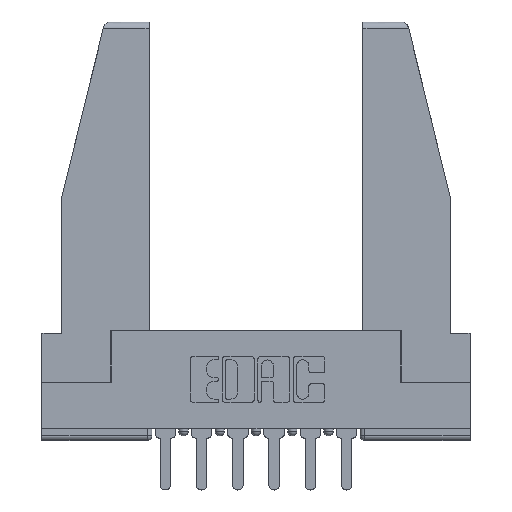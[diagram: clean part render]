
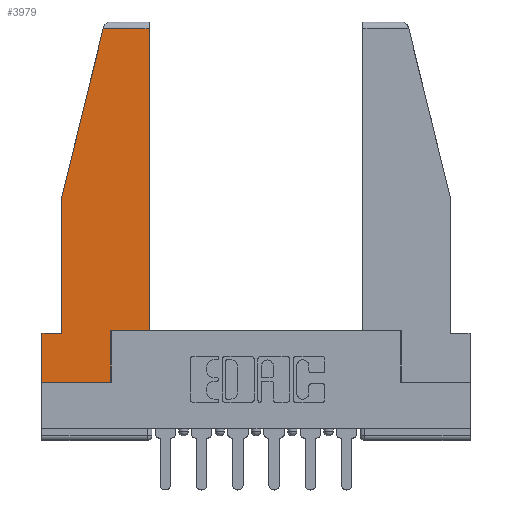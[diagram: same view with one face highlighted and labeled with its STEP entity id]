
A CAD part, top view. The second image highlights one B-rep face of the part: STEP entity #3979.
In plain terms, the highlighted planar face has unit normal (0, 0, 1).
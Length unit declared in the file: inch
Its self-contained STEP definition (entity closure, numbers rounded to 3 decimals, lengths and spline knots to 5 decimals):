
#81 = VERTEX_POINT ( 'NONE', #7556 ) ;
#235 = DIRECTION ( 'NONE',  ( 0., -1., 0. ) ) ;
#490 = LINE ( 'NONE', #7097, #2949 ) ;
#555 = CARTESIAN_POINT ( 'NONE',  ( 0.271, 1.55, 0. ) ) ;
#639 = CARTESIAN_POINT ( 'NONE',  ( 0.461, 1.52, 0. ) ) ;
#874 = EDGE_CURVE ( 'NONE', #11255, #3614, #11447, .T. ) ;
#1006 = ORIENTED_EDGE ( 'NONE', *, *, #5677, .T. ) ;
#1264 = CARTESIAN_POINT ( 'NONE',  ( 0.297, 0.223, 0. ) ) ;
#1443 = EDGE_CURVE ( 'NONE', #4556, #1515, #490, .T. ) ;
#1515 = VERTEX_POINT ( 'NONE', #9758 ) ;
#2089 = LINE ( 'NONE', #5869, #9575 ) ;
#2135 = ORIENTED_EDGE ( 'NONE', *, *, #4913, .T. ) ;
#2151 = VERTEX_POINT ( 'NONE', #10911 ) ;
#2249 = EDGE_CURVE ( 'NONE', #2151, #4882, #11339, .T. ) ;
#2949 = VECTOR ( 'NONE', #6114, 39.37008 ) ;
#2973 = FACE_OUTER_BOUND ( 'NONE', #5602, .T. ) ;
#3452 = CARTESIAN_POINT ( 'NONE',  ( 0.297, 0., 0. ) ) ;
#3614 = VERTEX_POINT ( 'NONE', #4164 ) ;
#3716 = ORIENTED_EDGE ( 'NONE', *, *, #8319, .T. ) ;
#3979 = ADVANCED_FACE ( 'NONE', ( #2973 ), #6754, .T. ) ;
#4010 = DIRECTION ( 'NONE',  ( -1., 0., 0. ) ) ;
#4101 = EDGE_CURVE ( 'NONE', #3614, #9369, #4502, .T. ) ;
#4164 = CARTESIAN_POINT ( 'NONE',  ( 0.297, 0., 0. ) ) ;
#4388 = VECTOR ( 'NONE', #10184, 39.37008 ) ;
#4502 = LINE ( 'NONE', #3452, #4388 ) ;
#4556 = VERTEX_POINT ( 'NONE', #639 ) ;
#4742 = ORIENTED_EDGE ( 'NONE', *, *, #8658, .T. ) ;
#4882 = VERTEX_POINT ( 'NONE', #7933 ) ;
#4913 = EDGE_CURVE ( 'NONE', #9369, #81, #5036, .T. ) ;
#4996 = CARTESIAN_POINT ( 'NONE',  ( 0., 0.21, 0. ) ) ;
#5036 = LINE ( 'NONE', #1264, #8338 ) ;
#5232 = CARTESIAN_POINT ( 'NONE',  ( 0.461, 0.223, 0. ) ) ;
#5293 = LINE ( 'NONE', #5232, #8551 ) ;
#5384 = ORIENTED_EDGE ( 'NONE', *, *, #2249, .T. ) ;
#5568 = DIRECTION ( 'NONE',  ( 0., 0., 1. ) ) ;
#5602 = EDGE_LOOP ( 'NONE', ( #1006, #5768, #3716, #5384, #4742, #7969, #5759, #8676, #2135 ) ) ;
#5677 = EDGE_CURVE ( 'NONE', #81, #4556, #5293, .T. ) ;
#5759 = ORIENTED_EDGE ( 'NONE', *, *, #874, .T. ) ;
#5768 = ORIENTED_EDGE ( 'NONE', *, *, #1443, .T. ) ;
#5784 = VECTOR ( 'NONE', #4010, 39.37008 ) ;
#5869 = CARTESIAN_POINT ( 'NONE',  ( 0., 0.21, 0. ) ) ;
#6114 = DIRECTION ( 'NONE',  ( -1., 0., 0. ) ) ;
#6341 = DIRECTION ( 'NONE',  ( 0., 1., 0. ) ) ;
#6673 = VECTOR ( 'NONE', #10585, 39.37008 ) ;
#6754 = PLANE ( 'NONE',  #10698 ) ;
#6773 = VECTOR ( 'NONE', #7278, 39.37008 ) ;
#7097 = CARTESIAN_POINT ( 'NONE',  ( 0., 1.52, 0. ) ) ;
#7278 = DIRECTION ( 'NONE',  ( -0.239, -0.971, 0. ) ) ;
#7556 = CARTESIAN_POINT ( 'NONE',  ( 0.461, 0.223, 0. ) ) ;
#7669 = CARTESIAN_POINT ( 'NONE',  ( 0., 0., 0. ) ) ;
#7713 = LINE ( 'NONE', #8689, #5784 ) ;
#7933 = CARTESIAN_POINT ( 'NONE',  ( 0.086, 0.21, 0. ) ) ;
#7969 = ORIENTED_EDGE ( 'NONE', *, *, #11056, .T. ) ;
#8082 = VECTOR ( 'NONE', #9461, 39.37008 ) ;
#8135 = LINE ( 'NONE', #555, #6773 ) ;
#8319 = EDGE_CURVE ( 'NONE', #1515, #2151, #8135, .T. ) ;
#8338 = VECTOR ( 'NONE', #8851, 39.37008 ) ;
#8401 = DIRECTION ( 'NONE',  ( 1., 0., 0. ) ) ;
#8551 = VECTOR ( 'NONE', #6341, 39.37008 ) ;
#8658 = EDGE_CURVE ( 'NONE', #4882, #11010, #7713, .T. ) ;
#8676 = ORIENTED_EDGE ( 'NONE', *, *, #4101, .T. ) ;
#8689 = CARTESIAN_POINT ( 'NONE',  ( 0., 0.21, 0. ) ) ;
#8851 = DIRECTION ( 'NONE',  ( 1., 0., 0. ) ) ;
#9369 = VERTEX_POINT ( 'NONE', #11744 ) ;
#9461 = DIRECTION ( 'NONE',  ( 0., -1., 0. ) ) ;
#9575 = VECTOR ( 'NONE', #235, 39.37008 ) ;
#9758 = CARTESIAN_POINT ( 'NONE',  ( 0.2636, 1.52, 0. ) ) ;
#10086 = CARTESIAN_POINT ( 'NONE',  ( 0., 0., 0. ) ) ;
#10184 = DIRECTION ( 'NONE',  ( 0., 1., 0. ) ) ;
#10250 = CARTESIAN_POINT ( 'NONE',  ( 0., 0., 0. ) ) ;
#10266 = CARTESIAN_POINT ( 'NONE',  ( 0.086, 0.8, 0. ) ) ;
#10585 = DIRECTION ( 'NONE',  ( 1., 0., 0. ) ) ;
#10698 = AXIS2_PLACEMENT_3D ( 'NONE', #10250, #5568, #8401 ) ;
#10911 = CARTESIAN_POINT ( 'NONE',  ( 0.086, 0.8, 0. ) ) ;
#11010 = VERTEX_POINT ( 'NONE', #4996 ) ;
#11056 = EDGE_CURVE ( 'NONE', #11010, #11255, #2089, .T. ) ;
#11255 = VERTEX_POINT ( 'NONE', #10086 ) ;
#11339 = LINE ( 'NONE', #10266, #8082 ) ;
#11447 = LINE ( 'NONE', #7669, #6673 ) ;
#11744 = CARTESIAN_POINT ( 'NONE',  ( 0.297, 0.223, 0. ) ) ;
